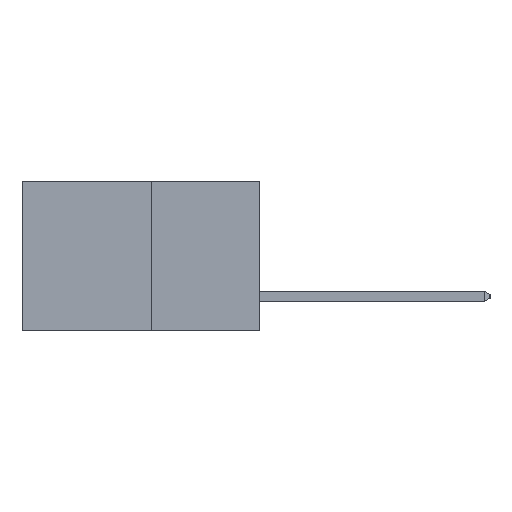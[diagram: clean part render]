
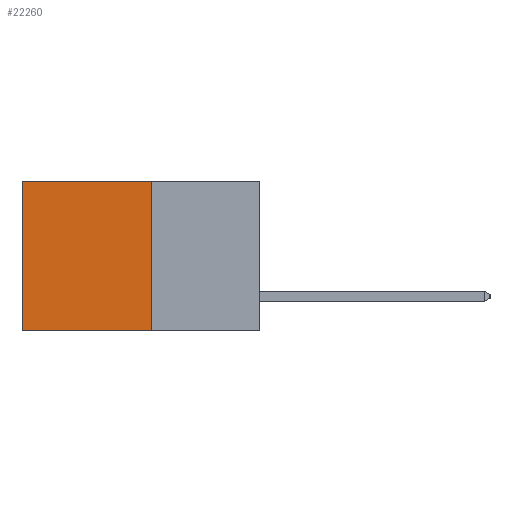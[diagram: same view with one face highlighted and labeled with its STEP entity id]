
A CAD part, left-side view. The second image highlights one B-rep face of the part: STEP entity #22260.
In plain terms, the highlighted planar face has unit normal (-1, 0, 0).
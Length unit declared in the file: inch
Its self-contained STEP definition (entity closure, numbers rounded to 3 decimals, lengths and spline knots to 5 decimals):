
#148 = DIRECTION ( 'NONE',  ( 0., 1., 0. ) ) ;
#366 = VERTEX_POINT ( 'NONE', #15280 ) ;
#809 = CARTESIAN_POINT ( 'NONE',  ( 0.277, 0.59, -0.37 ) ) ;
#946 = EDGE_CURVE ( 'NONE', #14735, #366, #6347, .T. ) ;
#1101 = VECTOR ( 'NONE', #148, 39.37008 ) ;
#3429 = PLANE ( 'NONE',  #5406 ) ;
#4540 = DIRECTION ( 'NONE',  ( 0., 0., -1. ) ) ;
#4720 = EDGE_CURVE ( 'NONE', #22764, #15591, #17627, .T. ) ;
#4967 = VECTOR ( 'NONE', #4540, 39.37008 ) ;
#5406 = AXIS2_PLACEMENT_3D ( 'NONE', #11174, #24204, #13063 ) ;
#6347 = LINE ( 'NONE', #15886, #1101 ) ;
#6450 = DIRECTION ( 'NONE',  ( 0., 1., 0. ) ) ;
#8391 = LINE ( 'NONE', #20699, #17768 ) ;
#9490 = LINE ( 'NONE', #15902, #4967 ) ;
#9866 = CARTESIAN_POINT ( 'NONE',  ( 0.277, 0.27, -0.37 ) ) ;
#11174 = CARTESIAN_POINT ( 'NONE',  ( 0.277, 0.27, -0.37 ) ) ;
#11416 = DIRECTION ( 'NONE',  ( 0., 0., -1. ) ) ;
#11628 = ORIENTED_EDGE ( 'NONE', *, *, #24578, .T. ) ;
#11745 = FACE_OUTER_BOUND ( 'NONE', #17710, .T. ) ;
#12686 = VECTOR ( 'NONE', #6450, 39.37008 ) ;
#13063 = DIRECTION ( 'NONE',  ( 0., 0., -1. ) ) ;
#14735 = VERTEX_POINT ( 'NONE', #24613 ) ;
#15280 = CARTESIAN_POINT ( 'NONE',  ( 0.277, 0.59, 0. ) ) ;
#15591 = VERTEX_POINT ( 'NONE', #809 ) ;
#15886 = CARTESIAN_POINT ( 'NONE',  ( 0.277, 0.27, 0. ) ) ;
#15902 = CARTESIAN_POINT ( 'NONE',  ( 0.277, 0.27, -0.37 ) ) ;
#17627 = LINE ( 'NONE', #9866, #12686 ) ;
#17710 = EDGE_LOOP ( 'NONE', ( #11628, #20374, #22716, #20667 ) ) ;
#17768 = VECTOR ( 'NONE', #11416, 39.37008 ) ;
#20122 = CARTESIAN_POINT ( 'NONE',  ( 0.277, 0.27, -0.37 ) ) ;
#20374 = ORIENTED_EDGE ( 'NONE', *, *, #4720, .F. ) ;
#20667 = ORIENTED_EDGE ( 'NONE', *, *, #946, .T. ) ;
#20699 = CARTESIAN_POINT ( 'NONE',  ( 0.277, 0.59, -0.37 ) ) ;
#20705 = EDGE_CURVE ( 'NONE', #14735, #22764, #9490, .T. ) ;
#22260 = ADVANCED_FACE ( 'NONE', ( #11745 ), #3429, .F. ) ;
#22716 = ORIENTED_EDGE ( 'NONE', *, *, #20705, .F. ) ;
#22764 = VERTEX_POINT ( 'NONE', #20122 ) ;
#24204 = DIRECTION ( 'NONE',  ( 1., 0., 0. ) ) ;
#24578 = EDGE_CURVE ( 'NONE', #366, #15591, #8391, .T. ) ;
#24613 = CARTESIAN_POINT ( 'NONE',  ( 0.277, 0.27, 0. ) ) ;
